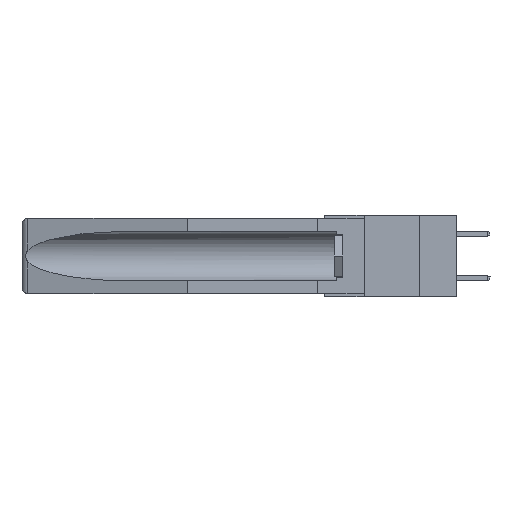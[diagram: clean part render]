
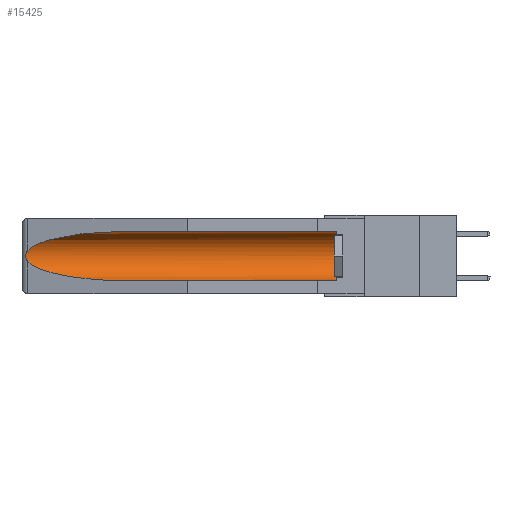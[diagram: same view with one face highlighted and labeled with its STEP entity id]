
A CAD part, left-side view. The second image highlights one B-rep face of the part: STEP entity #15425.
In plain terms, the highlighted cylindrical face has radius 2.857 mm (diameter 5.715 mm), a partial arc.
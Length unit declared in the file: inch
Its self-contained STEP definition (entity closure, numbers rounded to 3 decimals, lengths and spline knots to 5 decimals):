
#480 = CARTESIAN_POINT ( 'NONE',  ( 0.21114, 1.30732, -0.059 ) ) ;
#566 = ORIENTED_EDGE ( 'NONE', *, *, #12753, .F. ) ;
#1133 = CARTESIAN_POINT ( 'NONE',  ( 0.26537, 1.52718, -0.19328 ) ) ;
#1661 = DIRECTION ( 'NONE',  ( 0., -1., 0. ) ) ;
#1802 = CYLINDRICAL_SURFACE ( 'NONE', #15520, 0.1125 ) ;
#2605 = ORIENTED_EDGE ( 'NONE', *, *, #15789, .T. ) ;
#3140 = B_SPLINE_CURVE_WITH_KNOTS ( 'NONE', 3,
 ( #8103, #15792, #9617, #12575, #4978, #15714, #15638, #18700, #18628, #11133 ),
 .UNSPECIFIED., .F., .F.,
 ( 4, 2, 2, 2, 4 ),
 ( 0., 0.00029, 0.00058, 0.00087, 0.00117 ),
 .UNSPECIFIED. ) ;
#3172 = CIRCLE ( 'NONE', #18964, 0.1125 ) ;
#3434 = CARTESIAN_POINT ( 'NONE',  ( 0.26537, 1.52718, -0.14972 ) ) ;
#4462 = CARTESIAN_POINT ( 'NONE',  ( 0.155, 1.07973, -0.059 ) ) ;
#4978 = CARTESIAN_POINT ( 'NONE',  ( 0.2675, 1.53308, -0.16763 ) ) ;
#5600 = ORIENTED_EDGE ( 'NONE', *, *, #6487, .T. ) ;
#5767 = CARTESIAN_POINT ( 'NONE',  ( 0.155, 1.07973, -0.284 ) ) ;
#5995 = CARTESIAN_POINT ( 'NONE',  ( 0.155, 0.126, -0.059 ) ) ;
#6419 =( BOUNDED_CURVE ( )  B_SPLINE_CURVE ( 3, ( #17170, #9593, #18603, #6421 ),
 .UNSPECIFIED., .F., .F. ) 
 B_SPLINE_CURVE_WITH_KNOTS ( ( 4, 4 ),
 ( 0.1948, 1.5708 ),
 .UNSPECIFIED. ) 
 CURVE ( )  GEOMETRIC_REPRESENTATION_ITEM ( )  RATIONAL_B_SPLINE_CURVE ( ( 1., 0.848, 0.848, 1. ) ) 
 REPRESENTATION_ITEM ( '' )  );
#6421 = CARTESIAN_POINT ( 'NONE',  ( 0.155, 1.07973, -0.284 ) ) ;
#6487 = EDGE_CURVE ( 'NONE', #9920, #6792, #3172, .T. ) ;
#6496 = ORIENTED_EDGE ( 'NONE', *, *, #14533, .T. ) ;
#6724 = CARTESIAN_POINT ( 'NONE',  ( 0.155, 0.126, -0.1715 ) ) ;
#6780 = CARTESIAN_POINT ( 'NONE',  ( 0.155, 0.126, -0.284 ) ) ;
#6792 = VERTEX_POINT ( 'NONE', #5995 ) ;
#7703 = VECTOR ( 'NONE', #8136, 39.37008 ) ;
#7911 = DIRECTION ( 'NONE',  ( 0., 1., 0. ) ) ;
#8103 = CARTESIAN_POINT ( 'NONE',  ( 0.26537, 1.52718, -0.14972 ) ) ;
#8136 = DIRECTION ( 'NONE',  ( 0., 1., 0. ) ) ;
#9083 =( BOUNDED_CURVE ( )  B_SPLINE_CURVE ( 3, ( #17107, #480, #10921, #3434 ),
 .UNSPECIFIED., .F., .T. ) 
 B_SPLINE_CURVE_WITH_KNOTS ( ( 4, 4 ),
 ( 4.71239, 6.08839 ),
 .UNSPECIFIED. ) 
 CURVE ( )  GEOMETRIC_REPRESENTATION_ITEM ( )  RATIONAL_B_SPLINE_CURVE ( ( 1., 0.848, 0.848, 1. ) ) 
 REPRESENTATION_ITEM ( '' )  );
#9593 = CARTESIAN_POINT ( 'NONE',  ( 0.25451, 1.48313, -0.24835 ) ) ;
#9617 = CARTESIAN_POINT ( 'NONE',  ( 0.26654, 1.53092, -0.15636 ) ) ;
#9920 = VERTEX_POINT ( 'NONE', #6780 ) ;
#10002 = LINE ( 'NONE', #15716, #14962 ) ;
#10074 = ORIENTED_EDGE ( 'NONE', *, *, #10807, .T. ) ;
#10237 = CARTESIAN_POINT ( 'NONE',  ( 0.26537, 1.52718, -0.14972 ) ) ;
#10807 = EDGE_CURVE ( 'NONE', #6792, #14990, #19332, .T. ) ;
#10921 = CARTESIAN_POINT ( 'NONE',  ( 0.25451, 1.48313, -0.09465 ) ) ;
#11133 = CARTESIAN_POINT ( 'NONE',  ( 0.26537, 1.52718, -0.19328 ) ) ;
#11972 = CARTESIAN_POINT ( 'NONE',  ( 0.155, -0.30754, -0.1715 ) ) ;
#12098 = DIRECTION ( 'NONE',  ( 0., 1., 0. ) ) ;
#12123 = VERTEX_POINT ( 'NONE', #10237 ) ;
#12226 = FACE_OUTER_BOUND ( 'NONE', #15379, .T. ) ;
#12575 = CARTESIAN_POINT ( 'NONE',  ( 0.2673, 1.5327, -0.16383 ) ) ;
#12617 = CARTESIAN_POINT ( 'NONE',  ( 0.155, -0.30754, -0.059 ) ) ;
#12753 = EDGE_CURVE ( 'NONE', #9920, #15558, #10002, .T. ) ;
#14533 = EDGE_CURVE ( 'NONE', #12123, #15238, #3140, .T. ) ;
#14581 = ORIENTED_EDGE ( 'NONE', *, *, #14837, .T. ) ;
#14837 = EDGE_CURVE ( 'NONE', #15238, #15558, #6419, .T. ) ;
#14962 = VECTOR ( 'NONE', #7911, 39.37008 ) ;
#14990 = VERTEX_POINT ( 'NONE', #4462 ) ;
#15238 = VERTEX_POINT ( 'NONE', #1133 ) ;
#15379 = EDGE_LOOP ( 'NONE', ( #2605, #6496, #14581, #566, #5600, #10074 ) ) ;
#15425 = ADVANCED_FACE ( 'NONE', ( #12226 ), #1802, .F. ) ;
#15520 = AXIS2_PLACEMENT_3D ( 'NONE', #11972, #12098, #16855 ) ;
#15558 = VERTEX_POINT ( 'NONE', #5767 ) ;
#15638 = CARTESIAN_POINT ( 'NONE',  ( 0.2673, 1.53269, -0.17917 ) ) ;
#15714 = CARTESIAN_POINT ( 'NONE',  ( 0.2675, 1.53308, -0.17534 ) ) ;
#15716 = CARTESIAN_POINT ( 'NONE',  ( 0.155, -0.30754, -0.284 ) ) ;
#15789 = EDGE_CURVE ( 'NONE', #14990, #12123, #9083, .T. ) ;
#15792 = CARTESIAN_POINT ( 'NONE',  ( 0.26597, 1.52961, -0.15275 ) ) ;
#16855 = DIRECTION ( 'NONE',  ( 0., 0., 1. ) ) ;
#17107 = CARTESIAN_POINT ( 'NONE',  ( 0.155, 1.07973, -0.059 ) ) ;
#17170 = CARTESIAN_POINT ( 'NONE',  ( 0.26537, 1.52718, -0.19328 ) ) ;
#18603 = CARTESIAN_POINT ( 'NONE',  ( 0.21114, 1.30732, -0.284 ) ) ;
#18628 = CARTESIAN_POINT ( 'NONE',  ( 0.26597, 1.5296, -0.19026 ) ) ;
#18640 = DIRECTION ( 'NONE',  ( 0., 0., 1. ) ) ;
#18700 = CARTESIAN_POINT ( 'NONE',  ( 0.26655, 1.53094, -0.18657 ) ) ;
#18964 = AXIS2_PLACEMENT_3D ( 'NONE', #6724, #1661, #18640 ) ;
#19332 = LINE ( 'NONE', #12617, #7703 ) ;
